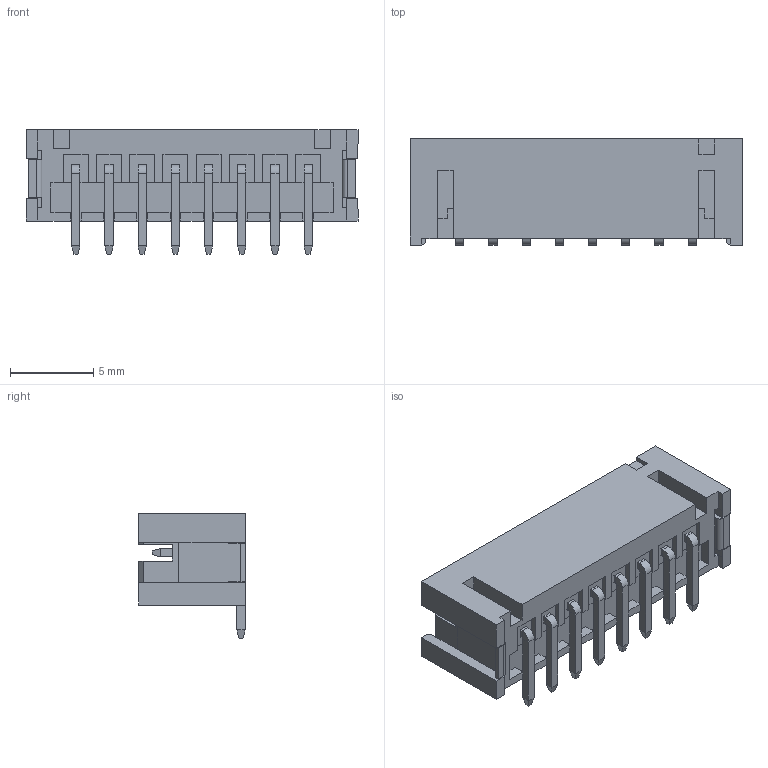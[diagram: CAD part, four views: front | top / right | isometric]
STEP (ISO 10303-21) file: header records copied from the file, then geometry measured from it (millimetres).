
FILE_DESCRIPTION (( 'STEP AP203' ), '1' );
FILE_NAME ('140-508-417-011.STEP', '2020-03-31T20:04:08', ( '' ), ( '' ), 'SwSTEP 2.0', 'SolidWorks 2016', '' );
FILE_SCHEMA (( 'CONFIG_CONTROL_DESIGN' ));
Length unit declared in the file: millimetre
Products named in the file (4): V SMT Contact; 140-508-417-011; V SMT Housing_508; V SMT Pad
Assembly tree (11 placements, depth 2):
  140-508-417-011
    V SMT Housing_508
    V SMT Contact  x8
    V SMT Pad  x2
Bounding box: 20 x 6.4 x 7.5 mm (x, y, z)
Volume: 299.8 mm3; surface area: 1079.7 mm2
Topology: 11 solids, 11 shells, 404 faces, 1020 edges, 634 vertices
Faces by surface type: plane 384, cylinder 20
Entity records: 8230 total; most frequent: CARTESIAN_POINT 1368, ORIENTED_EDGE 1352, DIRECTION 1184, EDGE_CURVE 676, VECTOR 668, LINE 668, VERTEX_POINT 442, AXIS2_PLACEMENT_3D 258
